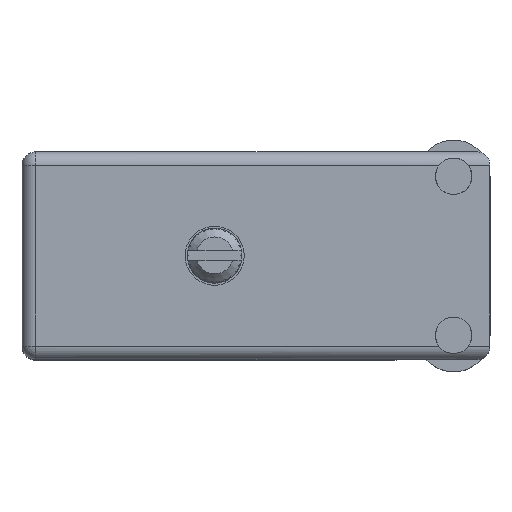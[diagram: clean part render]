
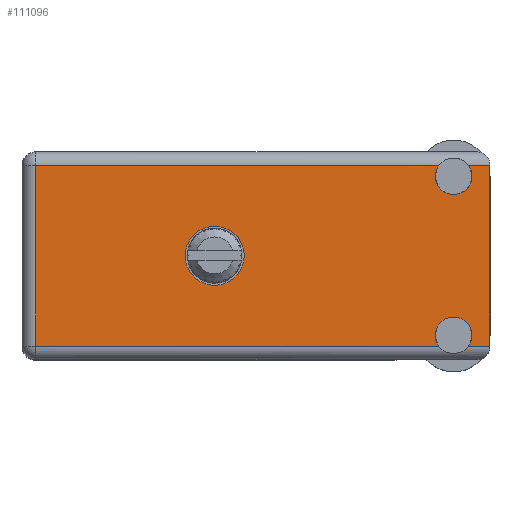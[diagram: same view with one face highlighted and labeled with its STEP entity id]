
A CAD part, top view. The second image highlights one B-rep face of the part: STEP entity #111096.
In plain terms, the highlighted face is planar.
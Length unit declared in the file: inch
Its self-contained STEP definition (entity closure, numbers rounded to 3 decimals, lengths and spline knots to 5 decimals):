
#1260 = CARTESIAN_POINT ( 'NONE',  ( 0.047, 0.906, -0.668 ) ) ;
#3703 = DIRECTION ( 'NONE',  ( 0., 1., 0. ) ) ;
#9201 = CARTESIAN_POINT ( 'NONE',  ( 0., 0.906, -0.715 ) ) ;
#15338 = CIRCLE ( 'NONE', #104033, 0.0625 ) ;
#18576 = CARTESIAN_POINT ( 'NONE',  ( 1.609, 0.906, -0.047 ) ) ;
#23198 = EDGE_CURVE ( 'NONE', #44532, #145716, #107408, .T. ) ;
#23688 = PLANE ( 'NONE',  #64684 ) ;
#23816 = DIRECTION ( 'NONE',  ( 0., 1., 0. ) ) ;
#25012 = CARTESIAN_POINT ( 'NONE',  ( 0., 0.906, -0.668 ) ) ;
#25811 = EDGE_CURVE ( 'NONE', #30068, #79615, #15338, .T. ) ;
#30068 = VERTEX_POINT ( 'NONE', #134760 ) ;
#32215 = ORIENTED_EDGE ( 'NONE', *, *, #164218, .F. ) ;
#33374 = CARTESIAN_POINT ( 'NONE',  ( 1.609, 0.906, -0.047 ) ) ;
#33851 = LINE ( 'NONE', #56505, #146810 ) ;
#33895 = ORIENTED_EDGE ( 'NONE', *, *, #141876, .F. ) ;
#34274 = EDGE_CURVE ( 'NONE', #151914, #82019, #33851, .T. ) ;
#34354 = ORIENTED_EDGE ( 'NONE', *, *, #110788, .F. ) ;
#38132 = AXIS2_PLACEMENT_3D ( 'NONE', #178214, #193430, #103222 ) ;
#39263 = VERTEX_POINT ( 'NONE', #1260 ) ;
#41979 = DIRECTION ( 'NONE',  ( -1., 0., 0. ) ) ;
#42620 = DIRECTION ( 'NONE',  ( 1., 0., 0. ) ) ;
#43273 = EDGE_CURVE ( 'NONE', #145716, #44532, #132780, .T. ) ;
#44532 = VERTEX_POINT ( 'NONE', #126786 ) ;
#47100 = CARTESIAN_POINT ( 'NONE',  ( 1.609, 0.906, -0.668 ) ) ;
#52064 = DIRECTION ( 'NONE',  ( 1., 0., 0. ) ) ;
#55680 = VECTOR ( 'NONE', #41979, 39.37008 ) ;
#55869 = CARTESIAN_POINT ( 'NONE',  ( 1.609, 0.906, 0. ) ) ;
#56505 = CARTESIAN_POINT ( 'NONE',  ( 1.609, 0.906, -0.047 ) ) ;
#59021 = VERTEX_POINT ( 'NONE', #145830 ) ;
#63554 = DIRECTION ( 'NONE',  ( 0., 0., 1. ) ) ;
#63986 = EDGE_CURVE ( 'NONE', #72634, #39263, #184743, .T. ) ;
#64684 = AXIS2_PLACEMENT_3D ( 'NONE', #9201, #157250, #69013 ) ;
#66188 = EDGE_CURVE ( 'NONE', #59021, #128188, #170206, .T. ) ;
#67189 = AXIS2_PLACEMENT_3D ( 'NONE', #74402, #147456, #192922 ) ;
#69013 = DIRECTION ( 'NONE',  ( 0., 0., 1. ) ) ;
#70408 = DIRECTION ( 'NONE',  ( 0., 0., 1. ) ) ;
#72007 = LINE ( 'NONE', #18576, #83929 ) ;
#72634 = VERTEX_POINT ( 'NONE', #93621 ) ;
#73650 = DIRECTION ( 'NONE',  ( -1., 0., 0. ) ) ;
#74402 = CARTESIAN_POINT ( 'NONE',  ( 0.6625, 0.906, -0.3575 ) ) ;
#77121 = CARTESIAN_POINT ( 'NONE',  ( 1.484, 0.906, -0.084 ) ) ;
#79615 = VERTEX_POINT ( 'NONE', #141804 ) ;
#81170 = CARTESIAN_POINT ( 'NONE',  ( 0.6625, 0.906, -0.256 ) ) ;
#82019 = VERTEX_POINT ( 'NONE', #33374 ) ;
#83929 = VECTOR ( 'NONE', #52064, 39.37008 ) ;
#93621 = CARTESIAN_POINT ( 'NONE',  ( 1.43363, 0.906, -0.668 ) ) ;
#94019 = CIRCLE ( 'NONE', #194922, 0.0625 ) ;
#95815 = ORIENTED_EDGE ( 'NONE', *, *, #43273, .F. ) ;
#97935 = ORIENTED_EDGE ( 'NONE', *, *, #34274, .T. ) ;
#99821 = EDGE_LOOP ( 'NONE', ( #95815, #190264 ) ) ;
#100761 = ORIENTED_EDGE ( 'NONE', *, *, #194266, .T. ) ;
#102447 = AXIS2_PLACEMENT_3D ( 'NONE', #172777, #3703, #63554 ) ;
#103222 = DIRECTION ( 'NONE',  ( 0., 0., 1. ) ) ;
#104033 = AXIS2_PLACEMENT_3D ( 'NONE', #173794, #23816, #128308 ) ;
#107408 = CIRCLE ( 'NONE', #67189, 0.1015 ) ;
#110788 = EDGE_CURVE ( 'NONE', #151914, #30068, #129894, .T. ) ;
#111096 = ADVANCED_FACE ( 'NONE', ( #179454, #139467 ), #23688, .T. ) ;
#111723 = ORIENTED_EDGE ( 'NONE', *, *, #63986, .T. ) ;
#113225 = CARTESIAN_POINT ( 'NONE',  ( 0.047, 0.906, -0.715 ) ) ;
#115905 = EDGE_LOOP ( 'NONE', ( #148000, #126446, #34354, #97935, #32215, #176725, #141599, #33895, #111723, #100761 ) ) ;
#122489 = DIRECTION ( 'NONE',  ( 0., 0., 1. ) ) ;
#123575 = EDGE_CURVE ( 'NONE', #136785, #79615, #72007, .T. ) ;
#124215 = DIRECTION ( 'NONE',  ( 0., 0., 1. ) ) ;
#126446 = ORIENTED_EDGE ( 'NONE', *, *, #25811, .F. ) ;
#126786 = CARTESIAN_POINT ( 'NONE',  ( 0.6625, 0.906, -0.459 ) ) ;
#128188 = VERTEX_POINT ( 'NONE', #152320 ) ;
#128308 = DIRECTION ( 'NONE',  ( 0., 0., 1. ) ) ;
#129894 = CIRCLE ( 'NONE', #155422, 0.0625 ) ;
#132780 = CIRCLE ( 'NONE', #38132, 0.1015 ) ;
#134285 = CARTESIAN_POINT ( 'NONE',  ( 1.53437, 0.906, -0.047 ) ) ;
#134760 = CARTESIAN_POINT ( 'NONE',  ( 1.484, 0.906, -0.1465 ) ) ;
#136138 = CARTESIAN_POINT ( 'NONE',  ( 0., 0.906, -0.668 ) ) ;
#136785 = VERTEX_POINT ( 'NONE', #177584 ) ;
#139467 = FACE_OUTER_BOUND ( 'NONE', #115905, .T. ) ;
#141599 = ORIENTED_EDGE ( 'NONE', *, *, #66188, .F. ) ;
#141804 = CARTESIAN_POINT ( 'NONE',  ( 1.43363, 0.906, -0.047 ) ) ;
#141876 = EDGE_CURVE ( 'NONE', #72634, #59021, #94019, .T. ) ;
#145716 = VERTEX_POINT ( 'NONE', #81170 ) ;
#145830 = CARTESIAN_POINT ( 'NONE',  ( 1.484, 0.906, -0.5685 ) ) ;
#146810 = VECTOR ( 'NONE', #42620, 39.37008 ) ;
#147456 = DIRECTION ( 'NONE',  ( 0., 1., 0. ) ) ;
#148000 = ORIENTED_EDGE ( 'NONE', *, *, #123575, .T. ) ;
#150744 = VERTEX_POINT ( 'NONE', #47100 ) ;
#151914 = VERTEX_POINT ( 'NONE', #134285 ) ;
#152085 = EDGE_CURVE ( 'NONE', #150744, #128188, #166532, .T. ) ;
#152320 = CARTESIAN_POINT ( 'NONE',  ( 1.53437, 0.906, -0.668 ) ) ;
#155422 = AXIS2_PLACEMENT_3D ( 'NONE', #77121, #182465, #122489 ) ;
#157250 = DIRECTION ( 'NONE',  ( 0., 1., 0. ) ) ;
#157718 = VECTOR ( 'NONE', #70408, 39.37008 ) ;
#164218 = EDGE_CURVE ( 'NONE', #150744, #82019, #187465, .T. ) ;
#164871 = LINE ( 'NONE', #113225, #157718 ) ;
#166532 = LINE ( 'NONE', #25012, #55680 ) ;
#169719 = DIRECTION ( 'NONE',  ( 0., 0., 1. ) ) ;
#170206 = CIRCLE ( 'NONE', #102447, 0.0625 ) ;
#172777 = CARTESIAN_POINT ( 'NONE',  ( 1.484, 0.906, -0.631 ) ) ;
#173294 = VECTOR ( 'NONE', #169719, 39.37008 ) ;
#173794 = CARTESIAN_POINT ( 'NONE',  ( 1.484, 0.906, -0.084 ) ) ;
#175216 = VECTOR ( 'NONE', #73650, 39.37008 ) ;
#176725 = ORIENTED_EDGE ( 'NONE', *, *, #152085, .T. ) ;
#177584 = CARTESIAN_POINT ( 'NONE',  ( 0.047, 0.906, -0.047 ) ) ;
#178214 = CARTESIAN_POINT ( 'NONE',  ( 0.6625, 0.906, -0.3575 ) ) ;
#179454 = FACE_BOUND ( 'NONE', #99821, .T. ) ;
#182465 = DIRECTION ( 'NONE',  ( 0., 1., 0. ) ) ;
#184743 = LINE ( 'NONE', #136138, #175216 ) ;
#184863 = DIRECTION ( 'NONE',  ( 0., 1., 0. ) ) ;
#185498 = CARTESIAN_POINT ( 'NONE',  ( 1.484, 0.906, -0.631 ) ) ;
#187465 = LINE ( 'NONE', #55869, #173294 ) ;
#190264 = ORIENTED_EDGE ( 'NONE', *, *, #23198, .F. ) ;
#192922 = DIRECTION ( 'NONE',  ( 0., 0., 1. ) ) ;
#193430 = DIRECTION ( 'NONE',  ( 0., 1., 0. ) ) ;
#194266 = EDGE_CURVE ( 'NONE', #39263, #136785, #164871, .T. ) ;
#194922 = AXIS2_PLACEMENT_3D ( 'NONE', #185498, #184863, #124215 ) ;
